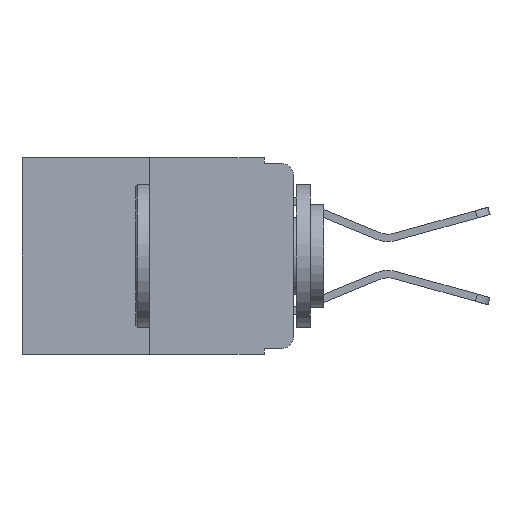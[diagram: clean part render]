
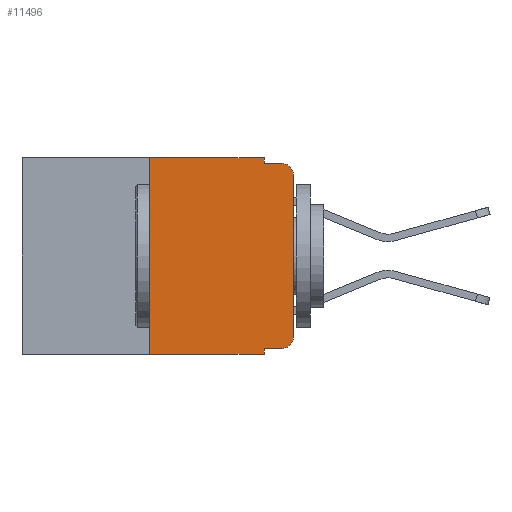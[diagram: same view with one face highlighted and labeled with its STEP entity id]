
A CAD part, left-side view. The second image highlights one B-rep face of the part: STEP entity #11496.
In plain terms, the highlighted planar face has unit normal (-1, 0, 0).
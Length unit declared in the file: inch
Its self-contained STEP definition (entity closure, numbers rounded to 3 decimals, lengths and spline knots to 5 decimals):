
#94 = EDGE_CURVE ( 'NONE', #9734, #7191, #150, .T. ) ;
#150 = LINE ( 'NONE', #5169, #11723 ) ;
#750 = CARTESIAN_POINT ( 'NONE',  ( 0., 0.02, -0.03 ) ) ;
#1337 = CARTESIAN_POINT ( 'NONE',  ( 0., 0.051, -0.01 ) ) ;
#1465 = AXIS2_PLACEMENT_3D ( 'NONE', #750, #9413, #9425 ) ;
#2000 = CARTESIAN_POINT ( 'NONE',  ( 0., 0.051, -0.333 ) ) ;
#2444 = VECTOR ( 'NONE', #17447, 39.37008 ) ;
#2839 = CIRCLE ( 'NONE', #16830, 0.02 ) ;
#2929 = LINE ( 'NONE', #5325, #17754 ) ;
#3052 = EDGE_CURVE ( 'NONE', #7191, #12608, #8772, .T. ) ;
#3446 = DIRECTION ( 'NONE',  ( -1., 0., 0. ) ) ;
#3652 = VECTOR ( 'NONE', #18472, 39.37008 ) ;
#3791 = ORIENTED_EDGE ( 'NONE', *, *, #13081, .T. ) ;
#4015 = CARTESIAN_POINT ( 'NONE',  ( 0., 0.473, 0. ) ) ;
#4046 = EDGE_CURVE ( 'NONE', #13992, #12608, #11604, .T. ) ;
#4541 = CARTESIAN_POINT ( 'NONE',  ( 0., 0., -0.313 ) ) ;
#4879 = VECTOR ( 'NONE', #15686, 39.37008 ) ;
#5169 = CARTESIAN_POINT ( 'NONE',  ( 0., 0.051, 0. ) ) ;
#5325 = CARTESIAN_POINT ( 'NONE',  ( 0., 0., 0. ) ) ;
#5612 = CARTESIAN_POINT ( 'NONE',  ( 0., 0.051, 0. ) ) ;
#5889 = CARTESIAN_POINT ( 'NONE',  ( 0., 0.473, 0. ) ) ;
#5995 = EDGE_CURVE ( 'NONE', #9193, #13992, #2929, .T. ) ;
#6640 = CARTESIAN_POINT ( 'NONE',  ( 0., 0.02, -0.01 ) ) ;
#6735 = ORIENTED_EDGE ( 'NONE', *, *, #16893, .F. ) ;
#6936 = DIRECTION ( 'NONE',  ( 0., 0., -1. ) ) ;
#7036 = VECTOR ( 'NONE', #9890, 39.37008 ) ;
#7191 = VERTEX_POINT ( 'NONE', #15394 ) ;
#7506 = CARTESIAN_POINT ( 'NONE',  ( 0., 0.25, -0.343 ) ) ;
#7525 = LINE ( 'NONE', #5612, #3652 ) ;
#7612 = ORIENTED_EDGE ( 'NONE', *, *, #5995, .T. ) ;
#7883 = CARTESIAN_POINT ( 'NONE',  ( 0., 0.25, 0. ) ) ;
#8396 = CARTESIAN_POINT ( 'NONE',  ( 0., 0., -0.03 ) ) ;
#8460 = CARTESIAN_POINT ( 'NONE',  ( 0., 0.25, 0. ) ) ;
#8556 = VERTEX_POINT ( 'NONE', #7506 ) ;
#8654 = FACE_OUTER_BOUND ( 'NONE', #9446, .T. ) ;
#8710 = VERTEX_POINT ( 'NONE', #7883 ) ;
#8772 = LINE ( 'NONE', #1337, #4879 ) ;
#8805 = ORIENTED_EDGE ( 'NONE', *, *, #18079, .T. ) ;
#8988 = ORIENTED_EDGE ( 'NONE', *, *, #4046, .T. ) ;
#9193 = VERTEX_POINT ( 'NONE', #4541 ) ;
#9375 = LINE ( 'NONE', #2000, #16044 ) ;
#9413 = DIRECTION ( 'NONE',  ( -1., 0., 0. ) ) ;
#9425 = DIRECTION ( 'NONE',  ( 0., 0., -1. ) ) ;
#9446 = EDGE_LOOP ( 'NONE', ( #7612, #8988, #12087, #12333, #11231, #15474, #8805, #6735, #14351, #3791 ) ) ;
#9707 = DIRECTION ( 'NONE',  ( 0., 0., 1. ) ) ;
#9734 = VERTEX_POINT ( 'NONE', #15703 ) ;
#9816 = VERTEX_POINT ( 'NONE', #15874 ) ;
#9890 = DIRECTION ( 'NONE',  ( 0., 0., 1. ) ) ;
#10981 = DIRECTION ( 'NONE',  ( 0., 0., -1. ) ) ;
#11231 = ORIENTED_EDGE ( 'NONE', *, *, #14166, .F. ) ;
#11450 = VERTEX_POINT ( 'NONE', #13942 ) ;
#11496 = ADVANCED_FACE ( 'NONE', ( #8654 ), #12642, .F. ) ;
#11604 = CIRCLE ( 'NONE', #1465, 0.02 ) ;
#11723 = VECTOR ( 'NONE', #10981, 39.37008 ) ;
#12082 = CARTESIAN_POINT ( 'NONE',  ( 0., 0.02, -0.313 ) ) ;
#12087 = ORIENTED_EDGE ( 'NONE', *, *, #3052, .F. ) ;
#12333 = ORIENTED_EDGE ( 'NONE', *, *, #94, .F. ) ;
#12608 = VERTEX_POINT ( 'NONE', #6640 ) ;
#12642 = PLANE ( 'NONE',  #14776 ) ;
#13081 = EDGE_CURVE ( 'NONE', #11450, #9193, #2839, .T. ) ;
#13507 = DIRECTION ( 'NONE',  ( 0., 0., -1. ) ) ;
#13942 = CARTESIAN_POINT ( 'NONE',  ( 0., 0.02, -0.333 ) ) ;
#13954 = LINE ( 'NONE', #16090, #2444 ) ;
#13992 = VERTEX_POINT ( 'NONE', #8396 ) ;
#14166 = EDGE_CURVE ( 'NONE', #8710, #9734, #14969, .T. ) ;
#14351 = ORIENTED_EDGE ( 'NONE', *, *, #15940, .T. ) ;
#14462 = DIRECTION ( 'NONE',  ( 0., -1., 0. ) ) ;
#14619 = LINE ( 'NONE', #8460, #7036 ) ;
#14776 = AXIS2_PLACEMENT_3D ( 'NONE', #4015, #15505, #6936 ) ;
#14897 = VERTEX_POINT ( 'NONE', #15533 ) ;
#14969 = LINE ( 'NONE', #5889, #18288 ) ;
#15394 = CARTESIAN_POINT ( 'NONE',  ( 0., 0.051, -0.01 ) ) ;
#15474 = ORIENTED_EDGE ( 'NONE', *, *, #17836, .F. ) ;
#15505 = DIRECTION ( 'NONE',  ( 1., 0., 0. ) ) ;
#15533 = CARTESIAN_POINT ( 'NONE',  ( 0., 0.051, -0.333 ) ) ;
#15686 = DIRECTION ( 'NONE',  ( 0., -1., 0. ) ) ;
#15703 = CARTESIAN_POINT ( 'NONE',  ( 0., 0.051, 0. ) ) ;
#15874 = CARTESIAN_POINT ( 'NONE',  ( 0., 0.051, -0.343 ) ) ;
#15940 = EDGE_CURVE ( 'NONE', #14897, #11450, #9375, .T. ) ;
#16044 = VECTOR ( 'NONE', #16433, 39.37008 ) ;
#16090 = CARTESIAN_POINT ( 'NONE',  ( 0., 0.473, -0.343 ) ) ;
#16433 = DIRECTION ( 'NONE',  ( 0., -1., 0. ) ) ;
#16830 = AXIS2_PLACEMENT_3D ( 'NONE', #12082, #3446, #13507 ) ;
#16893 = EDGE_CURVE ( 'NONE', #14897, #9816, #7525, .T. ) ;
#17447 = DIRECTION ( 'NONE',  ( 0., -1., 0. ) ) ;
#17754 = VECTOR ( 'NONE', #9707, 39.37008 ) ;
#17836 = EDGE_CURVE ( 'NONE', #8556, #8710, #14619, .T. ) ;
#18079 = EDGE_CURVE ( 'NONE', #8556, #9816, #13954, .T. ) ;
#18288 = VECTOR ( 'NONE', #14462, 39.37008 ) ;
#18472 = DIRECTION ( 'NONE',  ( 0., 0., -1. ) ) ;
